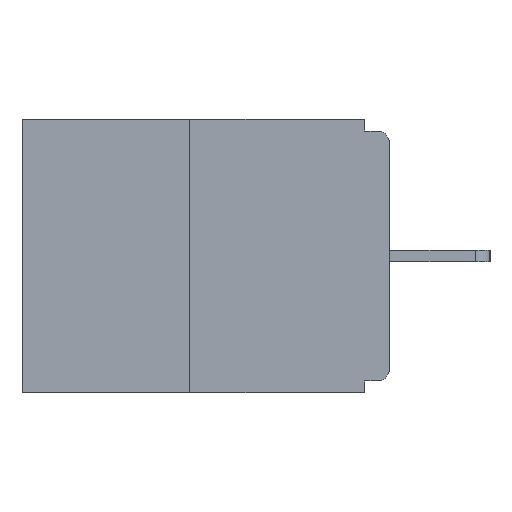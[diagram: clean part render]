
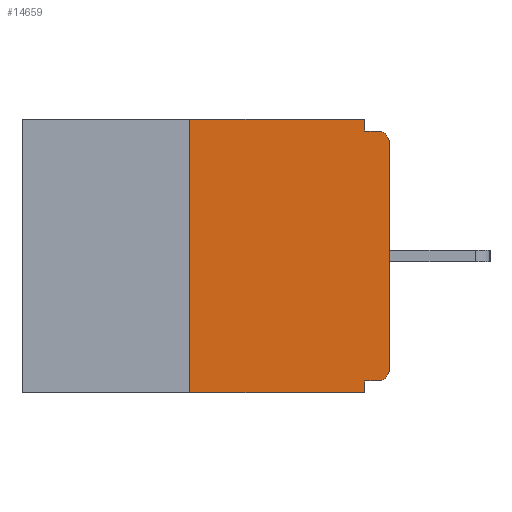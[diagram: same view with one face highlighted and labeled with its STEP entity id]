
A CAD part, left-side view. The second image highlights one B-rep face of the part: STEP entity #14659.
In plain terms, the highlighted planar face has unit normal (-1, 0, 0).
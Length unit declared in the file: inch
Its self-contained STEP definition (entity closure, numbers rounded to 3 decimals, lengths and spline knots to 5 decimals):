
#213 = CARTESIAN_POINT ( 'NONE',  ( 0., 0.25, -0.343 ) ) ;
#475 = EDGE_CURVE ( 'NONE', #18650, #14121, #5749, .T. ) ;
#617 = EDGE_CURVE ( 'NONE', #7011, #14121, #11273, .T. ) ;
#787 = VECTOR ( 'NONE', #3747, 39.37008 ) ;
#872 = CARTESIAN_POINT ( 'NONE',  ( 0., 0.031, -0.015 ) ) ;
#1198 = DIRECTION ( 'NONE',  ( -1., 0., 0. ) ) ;
#1695 = CARTESIAN_POINT ( 'NONE',  ( 0., 0.015, -0.03 ) ) ;
#1996 = VERTEX_POINT ( 'NONE', #11636 ) ;
#2057 = LINE ( 'NONE', #14343, #16779 ) ;
#2424 = VERTEX_POINT ( 'NONE', #15610 ) ;
#2777 = EDGE_CURVE ( 'NONE', #15737, #9753, #9302, .T. ) ;
#2908 = VECTOR ( 'NONE', #14649, 39.37008 ) ;
#2937 = AXIS2_PLACEMENT_3D ( 'NONE', #12384, #8067, #18116 ) ;
#3201 = LINE ( 'NONE', #17611, #6784 ) ;
#3219 = DIRECTION ( 'NONE',  ( 0., 0., -1. ) ) ;
#3224 = VERTEX_POINT ( 'NONE', #16221 ) ;
#3335 = VECTOR ( 'NONE', #7775, 39.37008 ) ;
#3462 = PLANE ( 'NONE',  #2937 ) ;
#3589 = EDGE_LOOP ( 'NONE', ( #18640, #18186, #9597, #17120, #9383, #18150, #16610, #18582, #4217, #18759 ) ) ;
#3747 = DIRECTION ( 'NONE',  ( 0., 0., -1. ) ) ;
#3834 = CARTESIAN_POINT ( 'NONE',  ( 0., 0.031, -0.343 ) ) ;
#4053 = DIRECTION ( 'NONE',  ( 0., -1., 0. ) ) ;
#4217 = ORIENTED_EDGE ( 'NONE', *, *, #18525, .F. ) ;
#5749 = LINE ( 'NONE', #11930, #16872 ) ;
#5837 = AXIS2_PLACEMENT_3D ( 'NONE', #1695, #12120, #3219 ) ;
#6090 = DIRECTION ( 'NONE',  ( 0., -1., 0. ) ) ;
#6784 = VECTOR ( 'NONE', #11917, 39.37008 ) ;
#7011 = VERTEX_POINT ( 'NONE', #8426 ) ;
#7064 = VERTEX_POINT ( 'NONE', #8068 ) ;
#7270 = DIRECTION ( 'NONE',  ( 0., 1., 0. ) ) ;
#7775 = DIRECTION ( 'NONE',  ( 0., 0., -1. ) ) ;
#8054 = VECTOR ( 'NONE', #7270, 39.37008 ) ;
#8067 = DIRECTION ( 'NONE',  ( 1., 0., 0. ) ) ;
#8068 = CARTESIAN_POINT ( 'NONE',  ( 0., 0.015, -0.015 ) ) ;
#8086 = EDGE_CURVE ( 'NONE', #3224, #16523, #18958, .T. ) ;
#8304 = VECTOR ( 'NONE', #13197, 39.37008 ) ;
#8426 = CARTESIAN_POINT ( 'NONE',  ( 0., 0.031, -0.328 ) ) ;
#8549 = EDGE_CURVE ( 'NONE', #2424, #15737, #2057, .T. ) ;
#8660 = CIRCLE ( 'NONE', #5837, 0.015 ) ;
#9302 = LINE ( 'NONE', #17497, #787 ) ;
#9383 = ORIENTED_EDGE ( 'NONE', *, *, #15477, .F. ) ;
#9430 = EDGE_CURVE ( 'NONE', #1996, #7064, #8660, .T. ) ;
#9597 = ORIENTED_EDGE ( 'NONE', *, *, #475, .T. ) ;
#9753 = VERTEX_POINT ( 'NONE', #872 ) ;
#9871 = CARTESIAN_POINT ( 'NONE',  ( 0., 0., -0.313 ) ) ;
#10230 = CARTESIAN_POINT ( 'NONE',  ( 0., 0.015, -0.313 ) ) ;
#10772 = CARTESIAN_POINT ( 'NONE',  ( 0., 0.031, 0. ) ) ;
#10847 = EDGE_CURVE ( 'NONE', #18650, #2424, #10875, .T. ) ;
#10875 = LINE ( 'NONE', #13246, #2908 ) ;
#11273 = LINE ( 'NONE', #3834, #3335 ) ;
#11636 = CARTESIAN_POINT ( 'NONE',  ( 0., 0., -0.03 ) ) ;
#11663 = DIRECTION ( 'NONE',  ( 0., 0., -1. ) ) ;
#11904 = LINE ( 'NONE', #14461, #8054 ) ;
#11917 = DIRECTION ( 'NONE',  ( 0., -1., 0. ) ) ;
#11930 = CARTESIAN_POINT ( 'NONE',  ( 0., 0.46, -0.343 ) ) ;
#12120 = DIRECTION ( 'NONE',  ( -1., 0., 0. ) ) ;
#12162 = LINE ( 'NONE', #14602, #8304 ) ;
#12384 = CARTESIAN_POINT ( 'NONE',  ( 0., 0.46, 0. ) ) ;
#13197 = DIRECTION ( 'NONE',  ( 0., 0., 1. ) ) ;
#13246 = CARTESIAN_POINT ( 'NONE',  ( 0., 0.25, 0. ) ) ;
#13961 = CARTESIAN_POINT ( 'NONE',  ( 0., 0.031, -0.343 ) ) ;
#14121 = VERTEX_POINT ( 'NONE', #13961 ) ;
#14343 = CARTESIAN_POINT ( 'NONE',  ( 0., 0.46, 0. ) ) ;
#14461 = CARTESIAN_POINT ( 'NONE',  ( 0., 0., -0.328 ) ) ;
#14602 = CARTESIAN_POINT ( 'NONE',  ( 0., 0., 0. ) ) ;
#14649 = DIRECTION ( 'NONE',  ( 0., 0., 1. ) ) ;
#14659 = ADVANCED_FACE ( 'NONE', ( #16637 ), #3462, .F. ) ;
#14897 = EDGE_CURVE ( 'NONE', #16523, #1996, #12162, .T. ) ;
#15161 = AXIS2_PLACEMENT_3D ( 'NONE', #10230, #1198, #11663 ) ;
#15477 = EDGE_CURVE ( 'NONE', #3224, #7011, #11904, .T. ) ;
#15610 = CARTESIAN_POINT ( 'NONE',  ( 0., 0.25, 0. ) ) ;
#15737 = VERTEX_POINT ( 'NONE', #10772 ) ;
#16221 = CARTESIAN_POINT ( 'NONE',  ( 0., 0.015, -0.328 ) ) ;
#16523 = VERTEX_POINT ( 'NONE', #9871 ) ;
#16610 = ORIENTED_EDGE ( 'NONE', *, *, #14897, .T. ) ;
#16637 = FACE_OUTER_BOUND ( 'NONE', #3589, .T. ) ;
#16779 = VECTOR ( 'NONE', #4053, 39.37008 ) ;
#16872 = VECTOR ( 'NONE', #6090, 39.37008 ) ;
#17120 = ORIENTED_EDGE ( 'NONE', *, *, #617, .F. ) ;
#17497 = CARTESIAN_POINT ( 'NONE',  ( 0., 0.031, 0. ) ) ;
#17611 = CARTESIAN_POINT ( 'NONE',  ( 0., 0., -0.015 ) ) ;
#18116 = DIRECTION ( 'NONE',  ( 0., 0., -1. ) ) ;
#18150 = ORIENTED_EDGE ( 'NONE', *, *, #8086, .T. ) ;
#18186 = ORIENTED_EDGE ( 'NONE', *, *, #10847, .F. ) ;
#18525 = EDGE_CURVE ( 'NONE', #9753, #7064, #3201, .T. ) ;
#18582 = ORIENTED_EDGE ( 'NONE', *, *, #9430, .T. ) ;
#18640 = ORIENTED_EDGE ( 'NONE', *, *, #8549, .F. ) ;
#18650 = VERTEX_POINT ( 'NONE', #213 ) ;
#18759 = ORIENTED_EDGE ( 'NONE', *, *, #2777, .F. ) ;
#18958 = CIRCLE ( 'NONE', #15161, 0.015 ) ;
